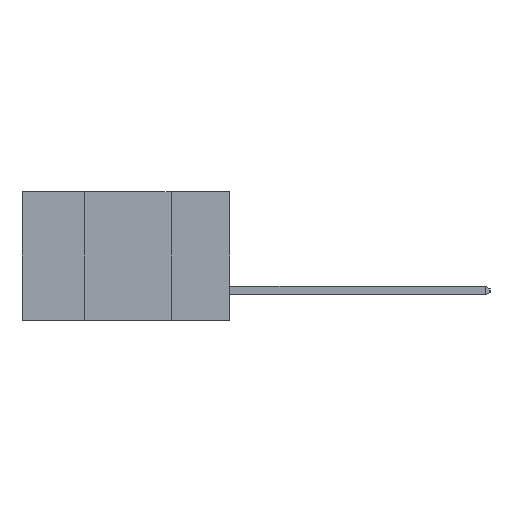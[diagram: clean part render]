
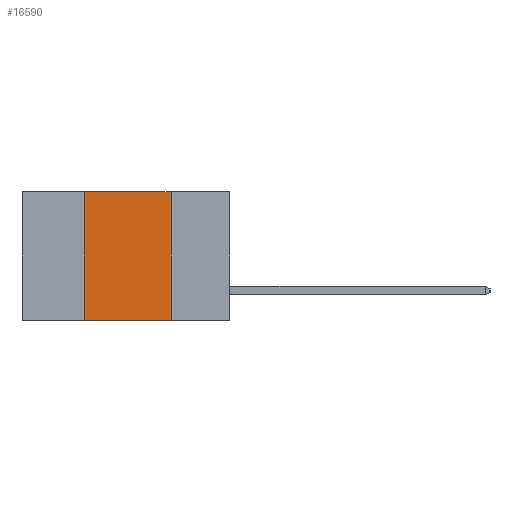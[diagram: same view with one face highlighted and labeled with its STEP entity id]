
A CAD part, left-side view. The second image highlights one B-rep face of the part: STEP entity #16590.
In plain terms, the highlighted planar face has unit normal (-1, 0, 0).
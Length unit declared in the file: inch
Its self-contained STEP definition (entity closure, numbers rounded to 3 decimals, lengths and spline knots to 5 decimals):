
#530 = DIRECTION ( 'NONE',  ( 0., -1., 0. ) ) ;
#663 = VERTEX_POINT ( 'NONE', #5513 ) ;
#1048 = CARTESIAN_POINT ( 'NONE',  ( 0., 0.42, 0. ) ) ;
#1164 = LINE ( 'NONE', #1048, #5730 ) ;
#2048 = LINE ( 'NONE', #24640, #11695 ) ;
#2140 = EDGE_CURVE ( 'NONE', #24765, #19571, #2048, .T. ) ;
#3180 = EDGE_LOOP ( 'NONE', ( #23775, #14602, #10747, #5915 ) ) ;
#3818 = DIRECTION ( 'NONE',  ( 1., 0., 0. ) ) ;
#5124 = CARTESIAN_POINT ( 'NONE',  ( 0., 0.17, -0.37 ) ) ;
#5372 = CARTESIAN_POINT ( 'NONE',  ( 0., 0.42, -0.37 ) ) ;
#5513 = CARTESIAN_POINT ( 'NONE',  ( 0., 0.42, 0. ) ) ;
#5730 = VECTOR ( 'NONE', #16465, 39.37008 ) ;
#5915 = ORIENTED_EDGE ( 'NONE', *, *, #17925, .T. ) ;
#5931 = EDGE_CURVE ( 'NONE', #663, #24765, #18435, .T. ) ;
#7760 = LINE ( 'NONE', #10174, #17379 ) ;
#10174 = CARTESIAN_POINT ( 'NONE',  ( 0., 0.6, -0.37 ) ) ;
#10425 = DIRECTION ( 'NONE',  ( 0., -1., 0. ) ) ;
#10747 = ORIENTED_EDGE ( 'NONE', *, *, #12258, .F. ) ;
#11239 = CARTESIAN_POINT ( 'NONE',  ( 0., 0.6, 0. ) ) ;
#11472 = CARTESIAN_POINT ( 'NONE',  ( 0., 0.6, 0. ) ) ;
#11695 = VECTOR ( 'NONE', #24955, 39.37008 ) ;
#12258 = EDGE_CURVE ( 'NONE', #17603, #663, #1164, .T. ) ;
#12409 = AXIS2_PLACEMENT_3D ( 'NONE', #11472, #3818, #17281 ) ;
#13280 = VECTOR ( 'NONE', #10425, 39.37008 ) ;
#14602 = ORIENTED_EDGE ( 'NONE', *, *, #5931, .F. ) ;
#16465 = DIRECTION ( 'NONE',  ( 0., 0., 1. ) ) ;
#16539 = CARTESIAN_POINT ( 'NONE',  ( 0., 0.17, 0. ) ) ;
#16590 = ADVANCED_FACE ( 'NONE', ( #18763 ), #22953, .F. ) ;
#17281 = DIRECTION ( 'NONE',  ( 0., 0., -1. ) ) ;
#17379 = VECTOR ( 'NONE', #530, 39.37008 ) ;
#17603 = VERTEX_POINT ( 'NONE', #5372 ) ;
#17925 = EDGE_CURVE ( 'NONE', #17603, #19571, #7760, .T. ) ;
#18435 = LINE ( 'NONE', #11239, #13280 ) ;
#18763 = FACE_OUTER_BOUND ( 'NONE', #3180, .T. ) ;
#19571 = VERTEX_POINT ( 'NONE', #5124 ) ;
#22953 = PLANE ( 'NONE',  #12409 ) ;
#23775 = ORIENTED_EDGE ( 'NONE', *, *, #2140, .F. ) ;
#24640 = CARTESIAN_POINT ( 'NONE',  ( 0., 0.17, 0. ) ) ;
#24765 = VERTEX_POINT ( 'NONE', #16539 ) ;
#24955 = DIRECTION ( 'NONE',  ( 0., 0., -1. ) ) ;
